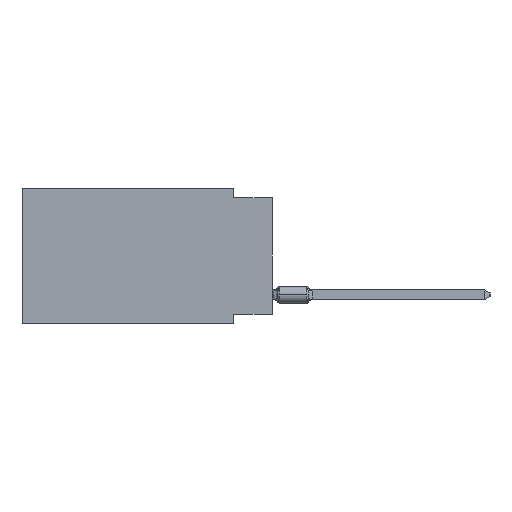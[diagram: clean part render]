
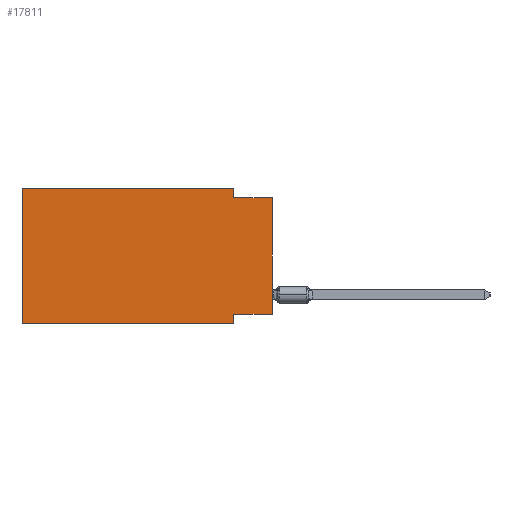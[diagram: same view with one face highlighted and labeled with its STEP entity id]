
A CAD part, left-side view. The second image highlights one B-rep face of the part: STEP entity #17811.
In plain terms, the highlighted planar face has unit normal (-1, 0, 0).
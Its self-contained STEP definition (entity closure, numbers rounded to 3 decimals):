
#632 = CARTESIAN_POINT ( 'NONE',  ( 0., 16.383, 0. ) ) ;
#682 = DIRECTION ( 'NONE',  ( 0., -1., 0. ) ) ;
#714 = CARTESIAN_POINT ( 'NONE',  ( 0., 16.383, -8.89 ) ) ;
#966 = CARTESIAN_POINT ( 'NONE',  ( 0., 2.54, 0. ) ) ;
#1283 = CARTESIAN_POINT ( 'NONE',  ( 0., 2.54, -8.255 ) ) ;
#1453 = CARTESIAN_POINT ( 'NONE',  ( 0., 2.54, -0.635 ) ) ;
#1782 = LINE ( 'NONE', #17442, #14762 ) ;
#2710 = CARTESIAN_POINT ( 'NONE',  ( 0., 0., 0. ) ) ;
#3098 = DIRECTION ( 'NONE',  ( 0., 0., -1. ) ) ;
#3123 = VECTOR ( 'NONE', #13981, 1000. ) ;
#3160 = CARTESIAN_POINT ( 'NONE',  ( 0., 0., -8.255 ) ) ;
#4748 = LINE ( 'NONE', #2710, #16853 ) ;
#5597 = ORIENTED_EDGE ( 'NONE', *, *, #32185, .T. ) ;
#5651 = CARTESIAN_POINT ( 'NONE',  ( 0., 2.54, -8.89 ) ) ;
#5997 = LINE ( 'NONE', #26374, #3123 ) ;
#7094 = EDGE_CURVE ( 'NONE', #26732, #17786, #1782, .T. ) ;
#7807 = DIRECTION ( 'NONE',  ( 0., 0., 1. ) ) ;
#8452 = FACE_OUTER_BOUND ( 'NONE', #32574, .T. ) ;
#8663 = CARTESIAN_POINT ( 'NONE',  ( 0., 16.383, 0. ) ) ;
#9592 = VECTOR ( 'NONE', #3098, 1000. ) ;
#10496 = VERTEX_POINT ( 'NONE', #21225 ) ;
#11013 = DIRECTION ( 'NONE',  ( 1., 0., 0. ) ) ;
#11016 = CARTESIAN_POINT ( 'NONE',  ( 0., 2.54, -8.89 ) ) ;
#13267 = EDGE_CURVE ( 'NONE', #28337, #26732, #27594, .T. ) ;
#13855 = EDGE_CURVE ( 'NONE', #25839, #27916, #25646, .T. ) ;
#13981 = DIRECTION ( 'NONE',  ( 0., -1., 0. ) ) ;
#14069 = VECTOR ( 'NONE', #29628, 1000. ) ;
#14176 = ORIENTED_EDGE ( 'NONE', *, *, #13267, .F. ) ;
#14468 = CARTESIAN_POINT ( 'NONE',  ( 0., 0., -0.635 ) ) ;
#14762 = VECTOR ( 'NONE', #30479, 1000. ) ;
#15991 = CARTESIAN_POINT ( 'NONE',  ( 0., 16.383, -8.89 ) ) ;
#16853 = VECTOR ( 'NONE', #28185, 1000. ) ;
#17315 = VECTOR ( 'NONE', #18124, 1000. ) ;
#17442 = CARTESIAN_POINT ( 'NONE',  ( 0., 0., -0.635 ) ) ;
#17786 = VERTEX_POINT ( 'NONE', #14468 ) ;
#17811 = ADVANCED_FACE ( 'NONE', ( #8452 ), #30738, .F. ) ;
#17950 = ORIENTED_EDGE ( 'NONE', *, *, #31202, .T. ) ;
#18124 = DIRECTION ( 'NONE',  ( 0., 1., 0. ) ) ;
#19621 = CARTESIAN_POINT ( 'NONE',  ( 0., 2.54, 0. ) ) ;
#19765 = ORIENTED_EDGE ( 'NONE', *, *, #23834, .F. ) ;
#20285 = EDGE_CURVE ( 'NONE', #22449, #25039, #28904, .T. ) ;
#20674 = LINE ( 'NONE', #3160, #17315 ) ;
#20953 = ORIENTED_EDGE ( 'NONE', *, *, #13855, .F. ) ;
#21017 = AXIS2_PLACEMENT_3D ( 'NONE', #632, #11013, #29158 ) ;
#21225 = CARTESIAN_POINT ( 'NONE',  ( 0., 0., -8.255 ) ) ;
#22449 = VERTEX_POINT ( 'NONE', #1283 ) ;
#23834 = EDGE_CURVE ( 'NONE', #10496, #22449, #20674, .T. ) ;
#25039 = VERTEX_POINT ( 'NONE', #11016 ) ;
#25217 = ORIENTED_EDGE ( 'NONE', *, *, #30581, .F. ) ;
#25646 = LINE ( 'NONE', #28680, #33061 ) ;
#25839 = VERTEX_POINT ( 'NONE', #714 ) ;
#26374 = CARTESIAN_POINT ( 'NONE',  ( 0., 16.383, 0. ) ) ;
#26732 = VERTEX_POINT ( 'NONE', #1453 ) ;
#27594 = LINE ( 'NONE', #19621, #14069 ) ;
#27916 = VERTEX_POINT ( 'NONE', #8663 ) ;
#28185 = DIRECTION ( 'NONE',  ( 0., 0., 1. ) ) ;
#28337 = VERTEX_POINT ( 'NONE', #966 ) ;
#28680 = CARTESIAN_POINT ( 'NONE',  ( 0., 16.383, 0. ) ) ;
#28808 = VECTOR ( 'NONE', #682, 1000. ) ;
#28904 = LINE ( 'NONE', #5651, #9592 ) ;
#29158 = DIRECTION ( 'NONE',  ( 0., 0., -1. ) ) ;
#29545 = LINE ( 'NONE', #15991, #28808 ) ;
#29628 = DIRECTION ( 'NONE',  ( 0., 0., -1. ) ) ;
#30479 = DIRECTION ( 'NONE',  ( 0., -1., 0. ) ) ;
#30581 = EDGE_CURVE ( 'NONE', #27916, #28337, #5997, .T. ) ;
#30738 = PLANE ( 'NONE',  #21017 ) ;
#31202 = EDGE_CURVE ( 'NONE', #10496, #17786, #4748, .T. ) ;
#31269 = ORIENTED_EDGE ( 'NONE', *, *, #20285, .F. ) ;
#32185 = EDGE_CURVE ( 'NONE', #25839, #25039, #29545, .T. ) ;
#32203 = ORIENTED_EDGE ( 'NONE', *, *, #7094, .F. ) ;
#32574 = EDGE_LOOP ( 'NONE', ( #17950, #32203, #14176, #25217, #20953, #5597, #31269, #19765 ) ) ;
#33061 = VECTOR ( 'NONE', #7807, 1000. ) ;
